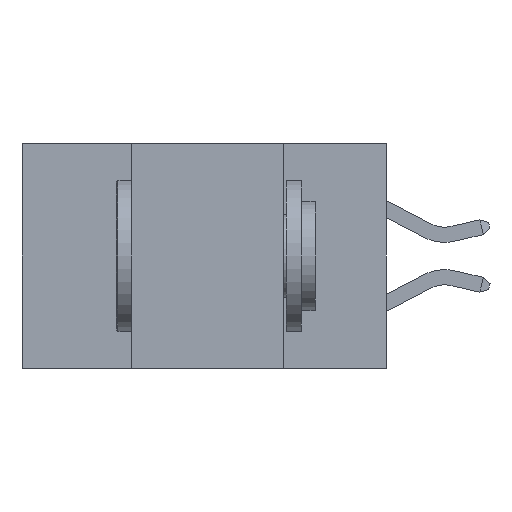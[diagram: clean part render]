
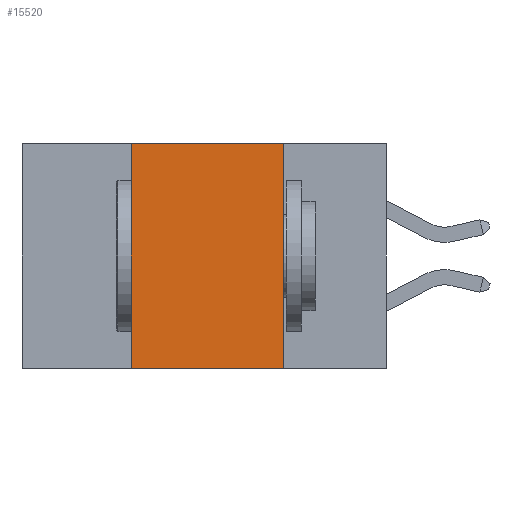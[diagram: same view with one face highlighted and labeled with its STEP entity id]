
A CAD part, left-side view. The second image highlights one B-rep face of the part: STEP entity #15520.
In plain terms, the highlighted planar face has unit normal (-1, 0, 0).
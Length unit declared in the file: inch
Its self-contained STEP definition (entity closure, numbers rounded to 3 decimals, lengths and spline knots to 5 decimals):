
#448 = DIRECTION ( 'NONE',  ( 1., 0., 0. ) ) ;
#548 = VECTOR ( 'NONE', #11261, 39.37008 ) ;
#1131 = EDGE_LOOP ( 'NONE', ( #15998, #17097, #3836, #8444 ) ) ;
#1133 = CARTESIAN_POINT ( 'NONE',  ( 0., 0.17, -0.37 ) ) ;
#1963 = AXIS2_PLACEMENT_3D ( 'NONE', #3875, #448, #12557 ) ;
#3148 = CARTESIAN_POINT ( 'NONE',  ( 0., 0.6, -0.37 ) ) ;
#3264 = CARTESIAN_POINT ( 'NONE',  ( 0., 0.42, -0.37 ) ) ;
#3438 = EDGE_CURVE ( 'NONE', #11890, #13903, #10306, .T. ) ;
#3471 = LINE ( 'NONE', #3148, #8067 ) ;
#3836 = ORIENTED_EDGE ( 'NONE', *, *, #11970, .F. ) ;
#3875 = CARTESIAN_POINT ( 'NONE',  ( 0., 0.6, 0. ) ) ;
#4588 = EDGE_CURVE ( 'NONE', #13903, #5691, #13499, .T. ) ;
#4604 = DIRECTION ( 'NONE',  ( 0., 0., -1. ) ) ;
#5691 = VERTEX_POINT ( 'NONE', #7357 ) ;
#7357 = CARTESIAN_POINT ( 'NONE',  ( 0., 0.17, -0.37 ) ) ;
#7468 = VECTOR ( 'NONE', #9907, 39.37008 ) ;
#8067 = VECTOR ( 'NONE', #13502, 39.37008 ) ;
#8444 = ORIENTED_EDGE ( 'NONE', *, *, #20093, .T. ) ;
#9458 = FACE_OUTER_BOUND ( 'NONE', #1131, .T. ) ;
#9907 = DIRECTION ( 'NONE',  ( 0., 0., 1. ) ) ;
#10306 = LINE ( 'NONE', #11306, #548 ) ;
#11261 = DIRECTION ( 'NONE',  ( 0., -1., 0. ) ) ;
#11306 = CARTESIAN_POINT ( 'NONE',  ( 0., 0.6, 0. ) ) ;
#11478 = CARTESIAN_POINT ( 'NONE',  ( 0., 0.42, 0. ) ) ;
#11767 = CARTESIAN_POINT ( 'NONE',  ( 0., 0.17, 0. ) ) ;
#11890 = VERTEX_POINT ( 'NONE', #11478 ) ;
#11970 = EDGE_CURVE ( 'NONE', #12049, #11890, #16678, .T. ) ;
#12049 = VERTEX_POINT ( 'NONE', #3264 ) ;
#12557 = DIRECTION ( 'NONE',  ( 0., 0., -1. ) ) ;
#13499 = LINE ( 'NONE', #1133, #22153 ) ;
#13502 = DIRECTION ( 'NONE',  ( 0., -1., 0. ) ) ;
#13903 = VERTEX_POINT ( 'NONE', #11767 ) ;
#15520 = ADVANCED_FACE ( 'NONE', ( #9458 ), #19442, .F. ) ;
#15998 = ORIENTED_EDGE ( 'NONE', *, *, #4588, .F. ) ;
#16678 = LINE ( 'NONE', #18610, #7468 ) ;
#17097 = ORIENTED_EDGE ( 'NONE', *, *, #3438, .F. ) ;
#18610 = CARTESIAN_POINT ( 'NONE',  ( 0., 0.42, -0.37 ) ) ;
#19442 = PLANE ( 'NONE',  #1963 ) ;
#20093 = EDGE_CURVE ( 'NONE', #12049, #5691, #3471, .T. ) ;
#22153 = VECTOR ( 'NONE', #4604, 39.37008 ) ;
